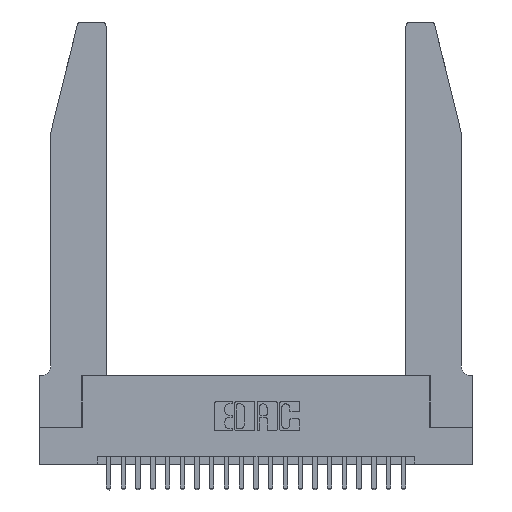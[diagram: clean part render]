
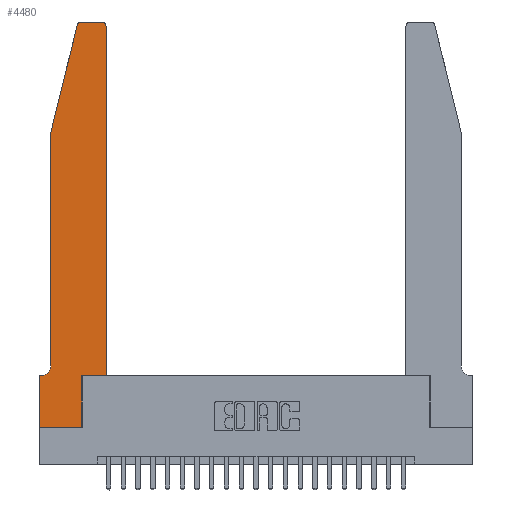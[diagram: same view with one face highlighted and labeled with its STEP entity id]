
A CAD part, top view. The second image highlights one B-rep face of the part: STEP entity #4480.
In plain terms, the highlighted planar face has unit normal (0, 0, 1).
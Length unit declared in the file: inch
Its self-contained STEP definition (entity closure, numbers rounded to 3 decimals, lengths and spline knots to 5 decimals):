
#980 = CARTESIAN_POINT ( 'NONE',  ( 0.4505, 0.35, 0.37 ) ) ;
#1046 = CARTESIAN_POINT ( 'NONE',  ( 0.284, 2.72, 0.37 ) ) ;
#1059 = EDGE_CURVE ( 'NONE', #3935, #1286, #10849, .T. ) ;
#1062 = VECTOR ( 'NONE', #3154, 39.37008 ) ;
#1286 = VERTEX_POINT ( 'NONE', #3255 ) ;
#1478 = CARTESIAN_POINT ( 'NONE',  ( 0., 0., 0.37 ) ) ;
#1850 = VECTOR ( 'NONE', #8522, 39.37008 ) ;
#2060 = VECTOR ( 'NONE', #7168, 39.37008 ) ;
#2305 = EDGE_CURVE ( 'NONE', #18535, #3764, #19239, .T. ) ;
#2696 = CARTESIAN_POINT ( 'NONE',  ( 0.4505, 2.72, 0.37 ) ) ;
#2799 = CARTESIAN_POINT ( 'NONE',  ( 0.2865, 0., 0.37 ) ) ;
#3022 = DIRECTION ( 'NONE',  ( 1., 0., 0. ) ) ;
#3154 = DIRECTION ( 'NONE',  ( 0., 1., 0. ) ) ;
#3192 = AXIS2_PLACEMENT_3D ( 'NONE', #20162, #9037, #21926 ) ;
#3255 = CARTESIAN_POINT ( 'NONE',  ( 0.0755, 0.42, 0.37 ) ) ;
#3270 = VECTOR ( 'NONE', #23764, 39.37008 ) ;
#3699 = EDGE_CURVE ( 'NONE', #7497, #11616, #4483, .T. ) ;
#3764 = VERTEX_POINT ( 'NONE', #13548 ) ;
#3765 = ORIENTED_EDGE ( 'NONE', *, *, #2305, .T. ) ;
#3935 = VERTEX_POINT ( 'NONE', #23001 ) ;
#4480 = ADVANCED_FACE ( 'NONE', ( #16851 ), #17689, .T. ) ;
#4483 = LINE ( 'NONE', #1478, #3270 ) ;
#4518 = EDGE_CURVE ( 'NONE', #3764, #8337, #10689, .T. ) ;
#4606 = DIRECTION ( 'NONE',  ( 0., 0., 1. ) ) ;
#4973 = VERTEX_POINT ( 'NONE', #19276 ) ;
#5707 = VERTEX_POINT ( 'NONE', #6119 ) ;
#6053 = LINE ( 'NONE', #10455, #10516 ) ;
#6119 = CARTESIAN_POINT ( 'NONE',  ( 0.284, 2.75, 0.37 ) ) ;
#6694 = ORIENTED_EDGE ( 'NONE', *, *, #22765, .T. ) ;
#7155 = CARTESIAN_POINT ( 'NONE',  ( 0.0755, 2., 0.37 ) ) ;
#7165 = EDGE_CURVE ( 'NONE', #7946, #5707, #6053, .T. ) ;
#7168 = DIRECTION ( 'NONE',  ( 0., -1., 0. ) ) ;
#7497 = VERTEX_POINT ( 'NONE', #22311 ) ;
#7792 = EDGE_LOOP ( 'NONE', ( #21390, #6694, #9458, #16164, #17410, #13677, #11514, #22512, #13798, #3765, #16527, #11446 ) ) ;
#7946 = VERTEX_POINT ( 'NONE', #9191 ) ;
#8031 = CARTESIAN_POINT ( 'NONE',  ( 0.0755, 0.35, 0.37 ) ) ;
#8337 = VERTEX_POINT ( 'NONE', #2696 ) ;
#8452 = EDGE_CURVE ( 'NONE', #4973, #3935, #23852, .T. ) ;
#8457 = AXIS2_PLACEMENT_3D ( 'NONE', #1046, #14458, #3022 ) ;
#8459 = AXIS2_PLACEMENT_3D ( 'NONE', #15943, #4606, #17772 ) ;
#8522 = DIRECTION ( 'NONE',  ( 0., -1., 0. ) ) ;
#8887 = VECTOR ( 'NONE', #13783, 39.37008 ) ;
#9037 = DIRECTION ( 'NONE',  ( 0., 0., -1. ) ) ;
#9191 = CARTESIAN_POINT ( 'NONE',  ( 0.4205, 2.75, 0.37 ) ) ;
#9273 = VECTOR ( 'NONE', #20201, 39.37008 ) ;
#9458 = ORIENTED_EDGE ( 'NONE', *, *, #8452, .T. ) ;
#10162 = EDGE_CURVE ( 'NONE', #12234, #15282, #24058, .T. ) ;
#10455 = CARTESIAN_POINT ( 'NONE',  ( 0.2605, 2.75, 0.37 ) ) ;
#10516 = VECTOR ( 'NONE', #19718, 39.37008 ) ;
#10688 = EDGE_CURVE ( 'NONE', #11616, #18535, #13670, .T. ) ;
#10689 = LINE ( 'NONE', #14569, #1062 ) ;
#10713 = EDGE_CURVE ( 'NONE', #8337, #7946, #22165, .T. ) ;
#10849 = LINE ( 'NONE', #13440, #1850 ) ;
#11328 = DIRECTION ( 'NONE',  ( 0., 0., 1. ) ) ;
#11446 = ORIENTED_EDGE ( 'NONE', *, *, #10713, .T. ) ;
#11514 = ORIENTED_EDGE ( 'NONE', *, *, #18359, .T. ) ;
#11611 = AXIS2_PLACEMENT_3D ( 'NONE', #22288, #11328, #24046 ) ;
#11616 = VERTEX_POINT ( 'NONE', #2799 ) ;
#12234 = VERTEX_POINT ( 'NONE', #21421 ) ;
#12847 = LINE ( 'NONE', #20212, #2060 ) ;
#13060 = VECTOR ( 'NONE', #23969, 39.37008 ) ;
#13088 = EDGE_CURVE ( 'NONE', #1286, #12234, #14981, .T. ) ;
#13440 = CARTESIAN_POINT ( 'NONE',  ( 0.0755, 2., 0.37 ) ) ;
#13548 = CARTESIAN_POINT ( 'NONE',  ( 0.4505, 0.35, 0.37 ) ) ;
#13670 = LINE ( 'NONE', #22216, #13060 ) ;
#13677 = ORIENTED_EDGE ( 'NONE', *, *, #10162, .T. ) ;
#13781 = VECTOR ( 'NONE', #18249, 39.37008 ) ;
#13783 = DIRECTION ( 'NONE',  ( -1., 0., 0. ) ) ;
#13798 = ORIENTED_EDGE ( 'NONE', *, *, #10688, .T. ) ;
#14458 = DIRECTION ( 'NONE',  ( 0., 0., 1. ) ) ;
#14569 = CARTESIAN_POINT ( 'NONE',  ( 0.4505, 0.35, 0.37 ) ) ;
#14981 = CIRCLE ( 'NONE', #3192, 0.07 ) ;
#15282 = VERTEX_POINT ( 'NONE', #20367 ) ;
#15943 = CARTESIAN_POINT ( 'NONE',  ( 0., 0.35, 0.37 ) ) ;
#16164 = ORIENTED_EDGE ( 'NONE', *, *, #1059, .T. ) ;
#16527 = ORIENTED_EDGE ( 'NONE', *, *, #4518, .T. ) ;
#16743 = CIRCLE ( 'NONE', #8457, 0.03 ) ;
#16851 = FACE_OUTER_BOUND ( 'NONE', #7792, .T. ) ;
#17410 = ORIENTED_EDGE ( 'NONE', *, *, #13088, .T. ) ;
#17689 = PLANE ( 'NONE',  #8459 ) ;
#17772 = DIRECTION ( 'NONE',  ( 1., 0., 0. ) ) ;
#18249 = DIRECTION ( 'NONE',  ( 1., 0., 0. ) ) ;
#18359 = EDGE_CURVE ( 'NONE', #15282, #7497, #12847, .T. ) ;
#18535 = VERTEX_POINT ( 'NONE', #18893 ) ;
#18893 = CARTESIAN_POINT ( 'NONE',  ( 0.2865, 0.35, 0.37 ) ) ;
#19239 = LINE ( 'NONE', #980, #13781 ) ;
#19276 = CARTESIAN_POINT ( 'NONE',  ( 0.25487, 2.72718, 0.37 ) ) ;
#19718 = DIRECTION ( 'NONE',  ( -1., 0., 0. ) ) ;
#20162 = CARTESIAN_POINT ( 'NONE',  ( 0.0055, 0.42, 0.37 ) ) ;
#20201 = DIRECTION ( 'NONE',  ( -0.239, -0.971, 0. ) ) ;
#20212 = CARTESIAN_POINT ( 'NONE',  ( 0., 0., 0.37 ) ) ;
#20367 = CARTESIAN_POINT ( 'NONE',  ( 0., 0.35, 0.37 ) ) ;
#21390 = ORIENTED_EDGE ( 'NONE', *, *, #7165, .T. ) ;
#21421 = CARTESIAN_POINT ( 'NONE',  ( 0.0055, 0.35, 0.37 ) ) ;
#21926 = DIRECTION ( 'NONE',  ( -1., 0., 0. ) ) ;
#22165 = CIRCLE ( 'NONE', #11611, 0.03 ) ;
#22216 = CARTESIAN_POINT ( 'NONE',  ( 0.2865, 0.35, 0.37 ) ) ;
#22288 = CARTESIAN_POINT ( 'NONE',  ( 0.4205, 2.72, 0.37 ) ) ;
#22311 = CARTESIAN_POINT ( 'NONE',  ( 0., 0., 0.37 ) ) ;
#22512 = ORIENTED_EDGE ( 'NONE', *, *, #3699, .T. ) ;
#22765 = EDGE_CURVE ( 'NONE', #5707, #4973, #16743, .T. ) ;
#23001 = CARTESIAN_POINT ( 'NONE',  ( 0.0755, 2., 0.37 ) ) ;
#23764 = DIRECTION ( 'NONE',  ( 1., 0., 0. ) ) ;
#23852 = LINE ( 'NONE', #7155, #9273 ) ;
#23969 = DIRECTION ( 'NONE',  ( 0., 1., 0. ) ) ;
#24046 = DIRECTION ( 'NONE',  ( 1., 0., 0. ) ) ;
#24058 = LINE ( 'NONE', #8031, #8887 ) ;
